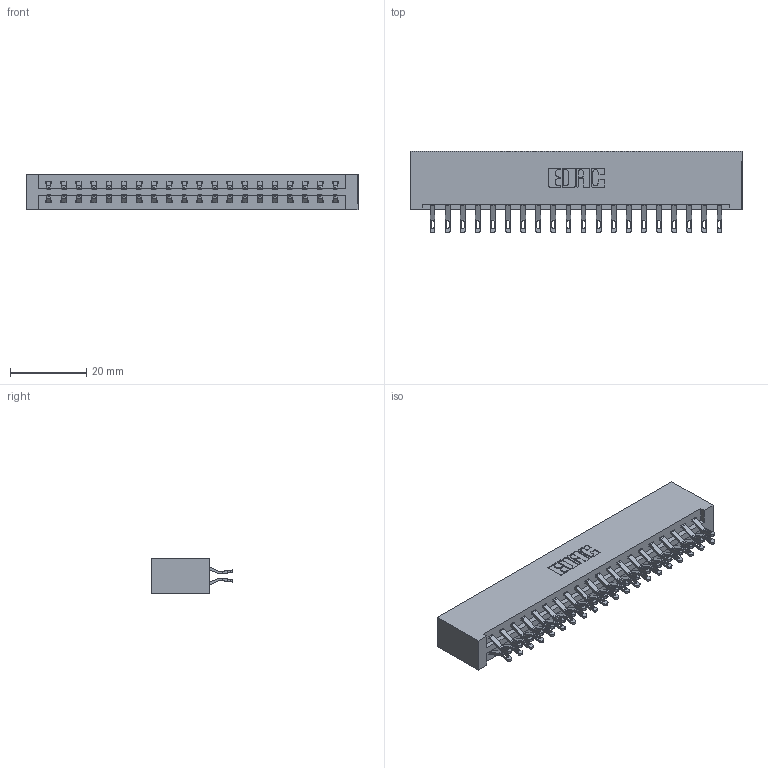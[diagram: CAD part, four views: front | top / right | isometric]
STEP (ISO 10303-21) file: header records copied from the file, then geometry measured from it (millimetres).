
FILE_DESCRIPTION (( 'STEP AP203' ), '1' );
FILE_NAME ('387-040-555-201.STEP', '2018-09-19T16:49:07', ( '' ), ( '' ), 'SwSTEP 2.0', 'SolidWorks 2016', '' );
FILE_SCHEMA (( 'CONFIG_CONTROL_DESIGN' ));
Length unit declared in the file: inch
Products named in the file (3): 337 Part_No Mounting Lugs; 345-292-001_555 Tail; 387-040-555-201
Assembly tree (41 placements, depth 2):
  387-040-555-201
    337 Part_No Mounting Lugs
    345-292-001_555 Tail  x40
Bounding box: 87.12 x 21.47 x 9.4 mm (x, y, z)
Volume: 9765.5 mm3; surface area: 11319.6 mm2
Topology: 41 solids, 41 shells, 2506 faces, 7847 edges, 5230 vertices
Faces by surface type: plane 1506, cylinder 1000
Entity records: 18401 total; most frequent: CARTESIAN_POINT 3152, ORIENTED_EDGE 3058, DIRECTION 2685, EDGE_CURVE 1529, LINE 1389, VECTOR 1389, VERTEX_POINT 1018, AXIS2_PLACEMENT_3D 648
